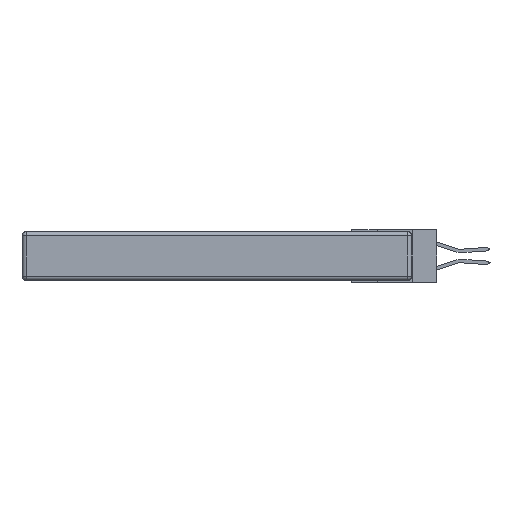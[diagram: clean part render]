
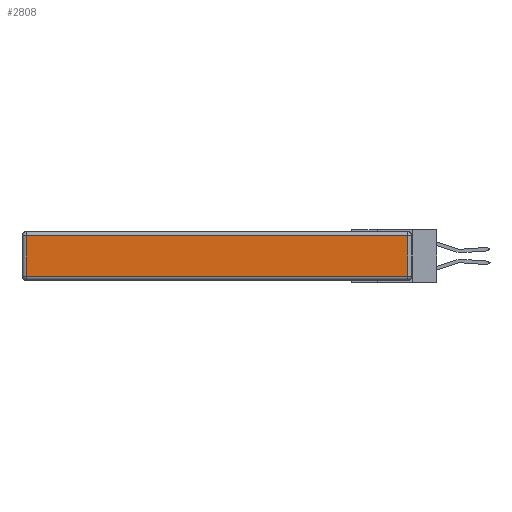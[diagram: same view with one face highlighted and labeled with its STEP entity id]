
A CAD part, left-side view. The second image highlights one B-rep face of the part: STEP entity #2808.
In plain terms, the highlighted planar face has unit normal (-1, 0, 0).
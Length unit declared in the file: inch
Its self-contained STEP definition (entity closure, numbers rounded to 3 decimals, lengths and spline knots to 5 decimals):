
#674 = CARTESIAN_POINT ( 'NONE',  ( 0., 0., -0.313 ) ) ;
#1171 = ORIENTED_EDGE ( 'NONE', *, *, #4104, .T. ) ;
#1576 = VECTOR ( 'NONE', #13858, 39.37008 ) ;
#2380 = FACE_OUTER_BOUND ( 'NONE', #21763, .T. ) ;
#2533 = VERTEX_POINT ( 'NONE', #4016 ) ;
#2775 = EDGE_CURVE ( 'NONE', #2533, #5428, #4232, .T. ) ;
#2782 = LINE ( 'NONE', #12310, #3140 ) ;
#2808 = ADVANCED_FACE ( 'NONE', ( #2380 ), #22965, .T. ) ;
#3140 = VECTOR ( 'NONE', #3148, 39.37008 ) ;
#3148 = DIRECTION ( 'NONE',  ( 0., 0., 1. ) ) ;
#3178 = CARTESIAN_POINT ( 'NONE',  ( 0., 2.72, -0.343 ) ) ;
#3201 = ORIENTED_EDGE ( 'NONE', *, *, #2775, .T. ) ;
#4016 = CARTESIAN_POINT ( 'NONE',  ( 0., 2.72, -0.03 ) ) ;
#4104 = EDGE_CURVE ( 'NONE', #17744, #2533, #19952, .T. ) ;
#4232 = LINE ( 'NONE', #3178, #21482 ) ;
#4786 = EDGE_CURVE ( 'NONE', #5428, #6234, #5227, .T. ) ;
#5227 = LINE ( 'NONE', #674, #14041 ) ;
#5428 = VERTEX_POINT ( 'NONE', #17131 ) ;
#5848 = CARTESIAN_POINT ( 'NONE',  ( 0., 0.03, -0.313 ) ) ;
#6234 = VERTEX_POINT ( 'NONE', #5848 ) ;
#9798 = AXIS2_PLACEMENT_3D ( 'NONE', #11403, #16035, #20738 ) ;
#11403 = CARTESIAN_POINT ( 'NONE',  ( 0., 0., -0.343 ) ) ;
#12310 = CARTESIAN_POINT ( 'NONE',  ( 0., 0.03, -0.343 ) ) ;
#13858 = DIRECTION ( 'NONE',  ( 0., 1., 0. ) ) ;
#14041 = VECTOR ( 'NONE', #19279, 39.37008 ) ;
#16035 = DIRECTION ( 'NONE',  ( -1., 0., 0. ) ) ;
#17131 = CARTESIAN_POINT ( 'NONE',  ( 0., 2.72, -0.313 ) ) ;
#17744 = VERTEX_POINT ( 'NONE', #22689 ) ;
#19279 = DIRECTION ( 'NONE',  ( 0., -1., 0. ) ) ;
#19952 = LINE ( 'NONE', #30145, #1576 ) ;
#20025 = EDGE_CURVE ( 'NONE', #6234, #17744, #2782, .T. ) ;
#20738 = DIRECTION ( 'NONE',  ( 0., 0., 1. ) ) ;
#21482 = VECTOR ( 'NONE', #30061, 39.37008 ) ;
#21763 = EDGE_LOOP ( 'NONE', ( #24268, #22890, #1171, #3201 ) ) ;
#22689 = CARTESIAN_POINT ( 'NONE',  ( 0., 0.03, -0.03 ) ) ;
#22890 = ORIENTED_EDGE ( 'NONE', *, *, #20025, .T. ) ;
#22965 = PLANE ( 'NONE',  #9798 ) ;
#24268 = ORIENTED_EDGE ( 'NONE', *, *, #4786, .T. ) ;
#30061 = DIRECTION ( 'NONE',  ( 0., 0., -1. ) ) ;
#30145 = CARTESIAN_POINT ( 'NONE',  ( 0., 2.75, -0.03 ) ) ;
